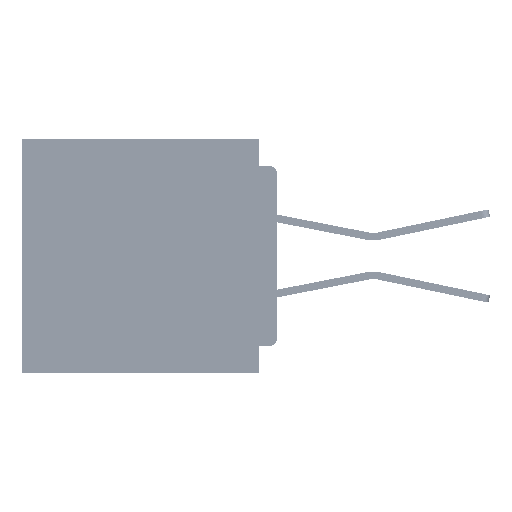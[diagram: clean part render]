
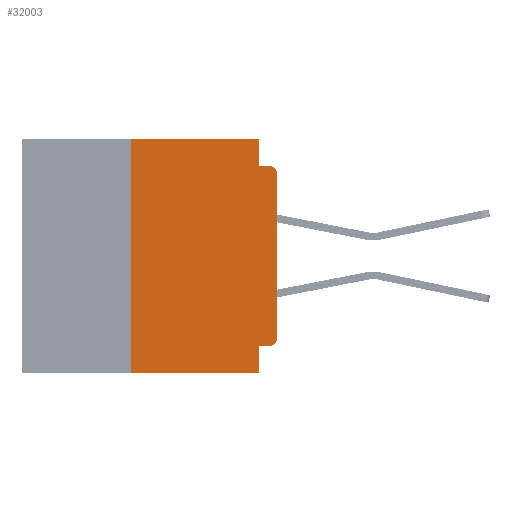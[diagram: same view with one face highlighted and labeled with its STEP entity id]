
A CAD part, left-side view. The second image highlights one B-rep face of the part: STEP entity #32003.
In plain terms, the highlighted planar face has unit normal (-1, 0, 0).
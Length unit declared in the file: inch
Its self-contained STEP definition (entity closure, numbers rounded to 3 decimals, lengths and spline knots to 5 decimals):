
#608 = CARTESIAN_POINT ( 'NONE',  ( 0., 0., -0.34 ) ) ;
#2970 = CARTESIAN_POINT ( 'NONE',  ( 0., 0.031, -0.4 ) ) ;
#6626 = CIRCLE ( 'NONE', #8644, 0.015 ) ;
#6658 = LINE ( 'NONE', #17539, #20703 ) ;
#8041 = DIRECTION ( 'NONE',  ( -1., 0., 0. ) ) ;
#8644 = AXIS2_PLACEMENT_3D ( 'NONE', #47773, #16082, #53052 ) ;
#9155 = VECTOR ( 'NONE', #35505, 39.37008 ) ;
#10441 = DIRECTION ( 'NONE',  ( 0., -1., 0. ) ) ;
#10810 = LINE ( 'NONE', #47004, #23244 ) ;
#13537 = CIRCLE ( 'NONE', #18236, 0.015 ) ;
#14447 = CARTESIAN_POINT ( 'NONE',  ( 0., 0.437, -0.4 ) ) ;
#14729 = CARTESIAN_POINT ( 'NONE',  ( 0., 0.031, 0. ) ) ;
#14960 = EDGE_CURVE ( 'NONE', #48613, #26093, #40645, .T. ) ;
#15386 = ORIENTED_EDGE ( 'NONE', *, *, #55127, .F. ) ;
#16082 = DIRECTION ( 'NONE',  ( -1., 0., 0. ) ) ;
#17467 = AXIS2_PLACEMENT_3D ( 'NONE', #54604, #49560, #17897 ) ;
#17539 = CARTESIAN_POINT ( 'NONE',  ( 0., 0.25, -0.4 ) ) ;
#17897 = DIRECTION ( 'NONE',  ( 0., 0., -1. ) ) ;
#18236 = AXIS2_PLACEMENT_3D ( 'NONE', #39766, #8041, #45028 ) ;
#18690 = LINE ( 'NONE', #55600, #59126 ) ;
#20703 = VECTOR ( 'NONE', #38575, 39.37008 ) ;
#20776 = DIRECTION ( 'NONE',  ( 0., -1., 0. ) ) ;
#20989 = CARTESIAN_POINT ( 'NONE',  ( 0., 0., -0.355 ) ) ;
#21235 = DIRECTION ( 'NONE',  ( 0., 0., -1. ) ) ;
#21562 = ORIENTED_EDGE ( 'NONE', *, *, #35131, .F. ) ;
#23033 = VECTOR ( 'NONE', #44723, 39.37008 ) ;
#23244 = VECTOR ( 'NONE', #10441, 39.37008 ) ;
#23488 = EDGE_CURVE ( 'NONE', #39405, #57245, #6626, .T. ) ;
#23679 = ORIENTED_EDGE ( 'NONE', *, *, #51896, .T. ) ;
#25237 = VERTEX_POINT ( 'NONE', #14729 ) ;
#26093 = VERTEX_POINT ( 'NONE', #2970 ) ;
#26870 = FACE_OUTER_BOUND ( 'NONE', #47848, .T. ) ;
#28655 = LINE ( 'NONE', #20989, #55020 ) ;
#30402 = EDGE_CURVE ( 'NONE', #36326, #61773, #28655, .T. ) ;
#31855 = VERTEX_POINT ( 'NONE', #608 ) ;
#32003 = ADVANCED_FACE ( 'NONE', ( #26870 ), #44237, .F. ) ;
#32331 = ORIENTED_EDGE ( 'NONE', *, *, #14960, .T. ) ;
#34627 = CARTESIAN_POINT ( 'NONE',  ( 0., 0.015, -0.045 ) ) ;
#34893 = CARTESIAN_POINT ( 'NONE',  ( 0., 0.015, -0.355 ) ) ;
#35131 = EDGE_CURVE ( 'NONE', #61773, #26093, #52807, .T. ) ;
#35252 = CARTESIAN_POINT ( 'NONE',  ( 0., 0.031, -0.045 ) ) ;
#35505 = DIRECTION ( 'NONE',  ( 0., -1., 0. ) ) ;
#36326 = VERTEX_POINT ( 'NONE', #34893 ) ;
#37761 = VERTEX_POINT ( 'NONE', #40692 ) ;
#37904 = EDGE_CURVE ( 'NONE', #37761, #25237, #57377, .T. ) ;
#38575 = DIRECTION ( 'NONE',  ( 0., 0., 1. ) ) ;
#39405 = VERTEX_POINT ( 'NONE', #54557 ) ;
#39766 = CARTESIAN_POINT ( 'NONE',  ( 0., 0.015, -0.34 ) ) ;
#40283 = VECTOR ( 'NONE', #21235, 39.37008 ) ;
#40645 = LINE ( 'NONE', #14447, #9155 ) ;
#40692 = CARTESIAN_POINT ( 'NONE',  ( 0., 0.25, 0. ) ) ;
#41008 = ORIENTED_EDGE ( 'NONE', *, *, #41516, .F. ) ;
#41516 = EDGE_CURVE ( 'NONE', #52656, #57245, #10810, .T. ) ;
#43347 = ORIENTED_EDGE ( 'NONE', *, *, #44471, .T. ) ;
#44237 = PLANE ( 'NONE',  #17467 ) ;
#44471 = EDGE_CURVE ( 'NONE', #31855, #39405, #18690, .T. ) ;
#44723 = DIRECTION ( 'NONE',  ( 0., 0., -1. ) ) ;
#45028 = DIRECTION ( 'NONE',  ( 0., 0., -1. ) ) ;
#46686 = VECTOR ( 'NONE', #20776, 39.37008 ) ;
#47004 = CARTESIAN_POINT ( 'NONE',  ( 0., 0., -0.045 ) ) ;
#47379 = CARTESIAN_POINT ( 'NONE',  ( 0., 0.437, 0. ) ) ;
#47773 = CARTESIAN_POINT ( 'NONE',  ( 0., 0.015, -0.06 ) ) ;
#47848 = EDGE_LOOP ( 'NONE', ( #43347, #61620, #41008, #15386, #52133, #51095, #32331, #21562, #68265, #23679 ) ) ;
#48613 = VERTEX_POINT ( 'NONE', #64112 ) ;
#49560 = DIRECTION ( 'NONE',  ( 1., 0., 0. ) ) ;
#50048 = CARTESIAN_POINT ( 'NONE',  ( 0., 0.031, -0.4 ) ) ;
#50337 = DIRECTION ( 'NONE',  ( 0., 0., 1. ) ) ;
#51095 = ORIENTED_EDGE ( 'NONE', *, *, #53693, .F. ) ;
#51896 = EDGE_CURVE ( 'NONE', #36326, #31855, #13537, .T. ) ;
#52133 = ORIENTED_EDGE ( 'NONE', *, *, #37904, .F. ) ;
#52656 = VERTEX_POINT ( 'NONE', #35252 ) ;
#52659 = DIRECTION ( 'NONE',  ( 0., 1., 0. ) ) ;
#52807 = LINE ( 'NONE', #50048, #23033 ) ;
#53052 = DIRECTION ( 'NONE',  ( 0., 0., -1. ) ) ;
#53117 = CARTESIAN_POINT ( 'NONE',  ( 0., 0.031, 0. ) ) ;
#53693 = EDGE_CURVE ( 'NONE', #48613, #37761, #6658, .T. ) ;
#54557 = CARTESIAN_POINT ( 'NONE',  ( 0., 0., -0.06 ) ) ;
#54604 = CARTESIAN_POINT ( 'NONE',  ( 0., 0.437, 0. ) ) ;
#55020 = VECTOR ( 'NONE', #52659, 39.37008 ) ;
#55127 = EDGE_CURVE ( 'NONE', #25237, #52656, #55908, .T. ) ;
#55600 = CARTESIAN_POINT ( 'NONE',  ( 0., 0., 0. ) ) ;
#55908 = LINE ( 'NONE', #53117, #40283 ) ;
#57245 = VERTEX_POINT ( 'NONE', #34627 ) ;
#57377 = LINE ( 'NONE', #47379, #46686 ) ;
#59126 = VECTOR ( 'NONE', #50337, 39.37008 ) ;
#61620 = ORIENTED_EDGE ( 'NONE', *, *, #23488, .T. ) ;
#61773 = VERTEX_POINT ( 'NONE', #68312 ) ;
#64112 = CARTESIAN_POINT ( 'NONE',  ( 0., 0.25, -0.4 ) ) ;
#68265 = ORIENTED_EDGE ( 'NONE', *, *, #30402, .F. ) ;
#68312 = CARTESIAN_POINT ( 'NONE',  ( 0., 0.031, -0.355 ) ) ;
